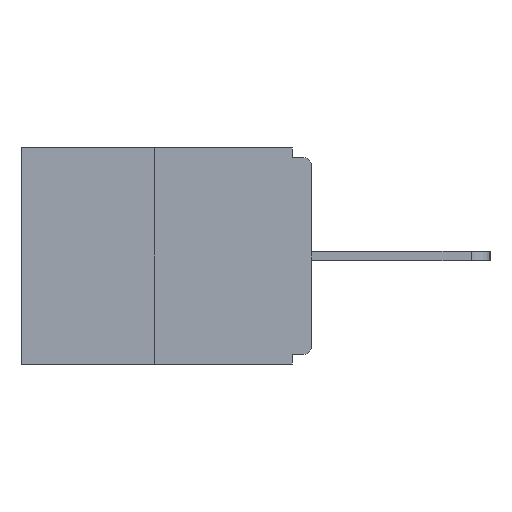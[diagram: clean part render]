
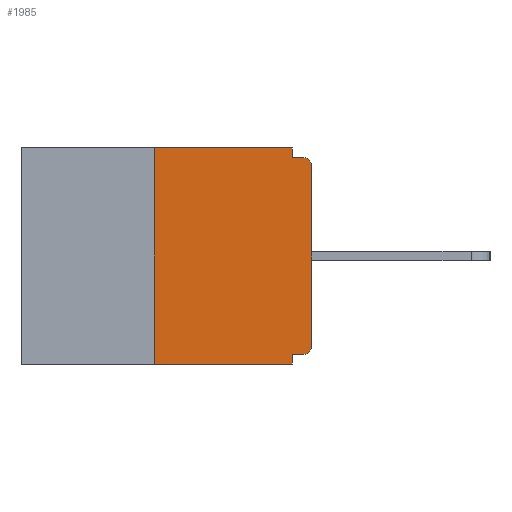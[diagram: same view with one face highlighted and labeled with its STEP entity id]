
A CAD part, left-side view. The second image highlights one B-rep face of the part: STEP entity #1985.
In plain terms, the highlighted planar face has unit normal (-1, 0, 0).
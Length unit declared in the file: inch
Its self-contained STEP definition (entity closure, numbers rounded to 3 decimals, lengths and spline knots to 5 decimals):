
#521 = VERTEX_POINT ( 'NONE', #14465 ) ;
#817 = CIRCLE ( 'NONE', #16977, 0.015 ) ;
#857 = VECTOR ( 'NONE', #14251, 39.37008 ) ;
#1377 = CARTESIAN_POINT ( 'NONE',  ( 0., 0.031, 0. ) ) ;
#1485 = VERTEX_POINT ( 'NONE', #17040 ) ;
#1524 = CARTESIAN_POINT ( 'NONE',  ( 0., 0.46, 0. ) ) ;
#1541 = CARTESIAN_POINT ( 'NONE',  ( 0., 0., 0. ) ) ;
#1585 = LINE ( 'NONE', #4299, #1799 ) ;
#1799 = VECTOR ( 'NONE', #18869, 39.37008 ) ;
#1940 = CIRCLE ( 'NONE', #10191, 0.015 ) ;
#1985 = ADVANCED_FACE ( 'NONE', ( #8994 ), #4511, .F. ) ;
#2153 = DIRECTION ( 'NONE',  ( 0., 0., -1. ) ) ;
#2810 = DIRECTION ( 'NONE',  ( 0., -1., 0. ) ) ;
#2991 = CARTESIAN_POINT ( 'NONE',  ( 0., 0., -0.328 ) ) ;
#3472 = CARTESIAN_POINT ( 'NONE',  ( 0., 0.25, 0. ) ) ;
#3870 = VECTOR ( 'NONE', #10522, 39.37008 ) ;
#4157 = VECTOR ( 'NONE', #4969, 39.37008 ) ;
#4299 = CARTESIAN_POINT ( 'NONE',  ( 0., 0.46, -0.343 ) ) ;
#4453 = EDGE_CURVE ( 'NONE', #14343, #7318, #14455, .T. ) ;
#4511 = PLANE ( 'NONE',  #9671 ) ;
#4572 = VECTOR ( 'NONE', #2153, 39.37008 ) ;
#4615 = DIRECTION ( 'NONE',  ( 0., 1., 0. ) ) ;
#4969 = DIRECTION ( 'NONE',  ( 0., 0., -1. ) ) ;
#4977 = DIRECTION ( 'NONE',  ( -1., 0., 0. ) ) ;
#4982 = CARTESIAN_POINT ( 'NONE',  ( 0., 0.031, -0.015 ) ) ;
#5102 = EDGE_CURVE ( 'NONE', #13036, #12356, #1940, .T. ) ;
#5423 = EDGE_LOOP ( 'NONE', ( #8842, #7024, #8178, #14597, #18624, #14928, #7427, #9594, #16704, #18577 ) ) ;
#5524 = VERTEX_POINT ( 'NONE', #15992 ) ;
#6221 = VECTOR ( 'NONE', #2810, 39.37008 ) ;
#6456 = EDGE_CURVE ( 'NONE', #16574, #14343, #17742, .T. ) ;
#7024 = ORIENTED_EDGE ( 'NONE', *, *, #7283, .F. ) ;
#7085 = DIRECTION ( 'NONE',  ( -1., 0., 0. ) ) ;
#7283 = EDGE_CURVE ( 'NONE', #521, #13064, #9121, .T. ) ;
#7287 = DIRECTION ( 'NONE',  ( 0., 0., -1. ) ) ;
#7318 = VERTEX_POINT ( 'NONE', #15104 ) ;
#7427 = ORIENTED_EDGE ( 'NONE', *, *, #12370, .T. ) ;
#7465 = CARTESIAN_POINT ( 'NONE',  ( 0., 0.031, 0. ) ) ;
#7947 = CARTESIAN_POINT ( 'NONE',  ( 0., 0.015, -0.313 ) ) ;
#8096 = LINE ( 'NONE', #13721, #4572 ) ;
#8178 = ORIENTED_EDGE ( 'NONE', *, *, #14969, .T. ) ;
#8638 = LINE ( 'NONE', #15582, #857 ) ;
#8771 = VECTOR ( 'NONE', #11767, 39.37008 ) ;
#8842 = ORIENTED_EDGE ( 'NONE', *, *, #14073, .F. ) ;
#8994 = FACE_OUTER_BOUND ( 'NONE', #5423, .T. ) ;
#9121 = LINE ( 'NONE', #3472, #3870 ) ;
#9198 = VERTEX_POINT ( 'NONE', #9841 ) ;
#9594 = ORIENTED_EDGE ( 'NONE', *, *, #12804, .T. ) ;
#9671 = AXIS2_PLACEMENT_3D ( 'NONE', #1524, #10314, #7287 ) ;
#9841 = CARTESIAN_POINT ( 'NONE',  ( 0., 0., -0.03 ) ) ;
#10191 = AXIS2_PLACEMENT_3D ( 'NONE', #7947, #4977, #17848 ) ;
#10314 = DIRECTION ( 'NONE',  ( 1., 0., 0. ) ) ;
#10522 = DIRECTION ( 'NONE',  ( 0., 0., 1. ) ) ;
#11353 = CARTESIAN_POINT ( 'NONE',  ( 0., 0.25, 0. ) ) ;
#11767 = DIRECTION ( 'NONE',  ( 0., 0., 1. ) ) ;
#12356 = VERTEX_POINT ( 'NONE', #17104 ) ;
#12370 = EDGE_CURVE ( 'NONE', #12356, #9198, #16250, .T. ) ;
#12382 = EDGE_CURVE ( 'NONE', #13036, #1485, #13301, .T. ) ;
#12804 = EDGE_CURVE ( 'NONE', #9198, #7318, #817, .T. ) ;
#13036 = VERTEX_POINT ( 'NONE', #15354 ) ;
#13064 = VERTEX_POINT ( 'NONE', #11353 ) ;
#13301 = LINE ( 'NONE', #2991, #13937 ) ;
#13721 = CARTESIAN_POINT ( 'NONE',  ( 0., 0.031, -0.343 ) ) ;
#13937 = VECTOR ( 'NONE', #4615, 39.37008 ) ;
#14073 = EDGE_CURVE ( 'NONE', #13064, #16574, #8638, .T. ) ;
#14251 = DIRECTION ( 'NONE',  ( 0., -1., 0. ) ) ;
#14343 = VERTEX_POINT ( 'NONE', #4982 ) ;
#14359 = CARTESIAN_POINT ( 'NONE',  ( 0., 0., -0.015 ) ) ;
#14455 = LINE ( 'NONE', #14359, #6221 ) ;
#14465 = CARTESIAN_POINT ( 'NONE',  ( 0., 0.25, -0.343 ) ) ;
#14597 = ORIENTED_EDGE ( 'NONE', *, *, #15152, .F. ) ;
#14789 = CARTESIAN_POINT ( 'NONE',  ( 0., 0.015, -0.03 ) ) ;
#14928 = ORIENTED_EDGE ( 'NONE', *, *, #5102, .T. ) ;
#14969 = EDGE_CURVE ( 'NONE', #521, #5524, #1585, .T. ) ;
#15104 = CARTESIAN_POINT ( 'NONE',  ( 0., 0.015, -0.015 ) ) ;
#15152 = EDGE_CURVE ( 'NONE', #1485, #5524, #8096, .T. ) ;
#15354 = CARTESIAN_POINT ( 'NONE',  ( 0., 0.015, -0.328 ) ) ;
#15582 = CARTESIAN_POINT ( 'NONE',  ( 0., 0.46, 0. ) ) ;
#15992 = CARTESIAN_POINT ( 'NONE',  ( 0., 0.031, -0.343 ) ) ;
#16250 = LINE ( 'NONE', #1541, #8771 ) ;
#16574 = VERTEX_POINT ( 'NONE', #1377 ) ;
#16704 = ORIENTED_EDGE ( 'NONE', *, *, #4453, .F. ) ;
#16977 = AXIS2_PLACEMENT_3D ( 'NONE', #14789, #7085, #17369 ) ;
#17040 = CARTESIAN_POINT ( 'NONE',  ( 0., 0.031, -0.328 ) ) ;
#17104 = CARTESIAN_POINT ( 'NONE',  ( 0., 0., -0.313 ) ) ;
#17369 = DIRECTION ( 'NONE',  ( 0., 0., -1. ) ) ;
#17742 = LINE ( 'NONE', #7465, #4157 ) ;
#17848 = DIRECTION ( 'NONE',  ( 0., 0., -1. ) ) ;
#18577 = ORIENTED_EDGE ( 'NONE', *, *, #6456, .F. ) ;
#18624 = ORIENTED_EDGE ( 'NONE', *, *, #12382, .F. ) ;
#18869 = DIRECTION ( 'NONE',  ( 0., -1., 0. ) ) ;
